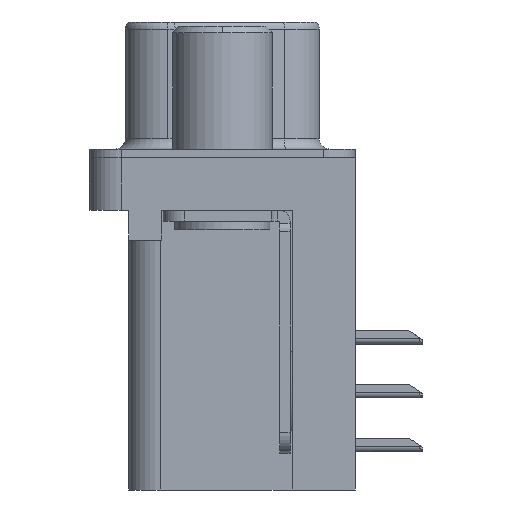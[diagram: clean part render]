
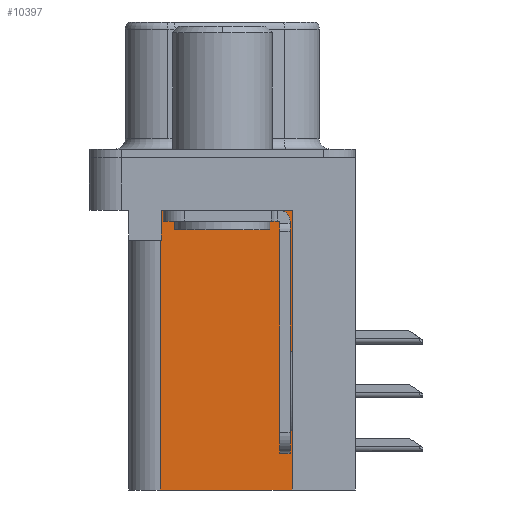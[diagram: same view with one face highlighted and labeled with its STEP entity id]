
A CAD part, left-side view. The second image highlights one B-rep face of the part: STEP entity #10397.
In plain terms, the highlighted planar face has unit normal (-1, 0, 0).
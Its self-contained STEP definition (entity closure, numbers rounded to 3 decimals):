
#514 = ORIENTED_EDGE ( 'NONE', *, *, #18524, .F. ) ;
#547 = DIRECTION ( 'NONE',  ( 0., 0., 1. ) ) ;
#1839 = ORIENTED_EDGE ( 'NONE', *, *, #3769, .T. ) ;
#2024 = CARTESIAN_POINT ( 'NONE',  ( 3.765, 2.895, -3.9 ) ) ;
#2810 = CARTESIAN_POINT ( 'NONE',  ( 3.765, -3.295, -2.5 ) ) ;
#2823 = CARTESIAN_POINT ( 'NONE',  ( 3.765, -3.295, -15.7 ) ) ;
#3165 = VERTEX_POINT ( 'NONE', #2810 ) ;
#3436 = VECTOR ( 'NONE', #25121, 1000. ) ;
#3769 = EDGE_CURVE ( 'NONE', #14060, #10398, #19271, .T. ) ;
#3882 = DIRECTION ( 'NONE',  ( 0., 0., -1. ) ) ;
#4667 = VERTEX_POINT ( 'NONE', #24077 ) ;
#4865 = VECTOR ( 'NONE', #547, 1000. ) ;
#5371 = VECTOR ( 'NONE', #24765, 1000. ) ;
#5867 = PLANE ( 'NONE',  #14750 ) ;
#6328 = EDGE_CURVE ( 'NONE', #3165, #4667, #23820, .T. ) ;
#6527 = ORIENTED_EDGE ( 'NONE', *, *, #6328, .T. ) ;
#6721 = VECTOR ( 'NONE', #19898, 1000. ) ;
#6760 = EDGE_CURVE ( 'NONE', #21742, #3165, #22274, .T. ) ;
#7051 = CARTESIAN_POINT ( 'NONE',  ( 3.765, 2.925, -15.7 ) ) ;
#7304 = VECTOR ( 'NONE', #22511, 1000. ) ;
#7611 = ORIENTED_EDGE ( 'NONE', *, *, #6760, .T. ) ;
#8208 = FACE_OUTER_BOUND ( 'NONE', #23082, .T. ) ;
#8701 = CARTESIAN_POINT ( 'NONE',  ( 3.765, -3.295, -15.7 ) ) ;
#9380 = VECTOR ( 'NONE', #25469, 1000. ) ;
#9716 = CARTESIAN_POINT ( 'NONE',  ( 3.765, -3.295, -15.7 ) ) ;
#10162 = EDGE_CURVE ( 'NONE', #21742, #13282, #22407, .T. ) ;
#10397 = ADVANCED_FACE ( 'NONE', ( #8208 ), #5867, .F. ) ;
#10398 = VERTEX_POINT ( 'NONE', #11663 ) ;
#10455 = CARTESIAN_POINT ( 'NONE',  ( 3.765, 2.925, -15.7 ) ) ;
#11663 = CARTESIAN_POINT ( 'NONE',  ( 3.765, 2.925, -3.9 ) ) ;
#13259 = CARTESIAN_POINT ( 'NONE',  ( 3.765, -3.295, -2.5 ) ) ;
#13282 = VERTEX_POINT ( 'NONE', #7051 ) ;
#14060 = VERTEX_POINT ( 'NONE', #14902 ) ;
#14750 = AXIS2_PLACEMENT_3D ( 'NONE', #9716, #15674, #3882 ) ;
#14902 = CARTESIAN_POINT ( 'NONE',  ( 3.765, 2.895, -3.9 ) ) ;
#15674 = DIRECTION ( 'NONE',  ( 1., 0., 0. ) ) ;
#17856 = EDGE_CURVE ( 'NONE', #4667, #14060, #22426, .T. ) ;
#18406 = ORIENTED_EDGE ( 'NONE', *, *, #17856, .T. ) ;
#18524 = EDGE_CURVE ( 'NONE', #13282, #10398, #20532, .T. ) ;
#19271 = LINE ( 'NONE', #23723, #9380 ) ;
#19898 = DIRECTION ( 'NONE',  ( 0., 0., -1. ) ) ;
#20532 = LINE ( 'NONE', #10455, #4865 ) ;
#21742 = VERTEX_POINT ( 'NONE', #2823 ) ;
#22274 = LINE ( 'NONE', #22783, #5371 ) ;
#22407 = LINE ( 'NONE', #8701, #7304 ) ;
#22426 = LINE ( 'NONE', #2024, #6721 ) ;
#22511 = DIRECTION ( 'NONE',  ( 0., 1., 0. ) ) ;
#22783 = CARTESIAN_POINT ( 'NONE',  ( 3.765, -3.295, -15.7 ) ) ;
#23082 = EDGE_LOOP ( 'NONE', ( #6527, #18406, #1839, #514, #23744, #7611 ) ) ;
#23723 = CARTESIAN_POINT ( 'NONE',  ( 3.765, 0., -3.9 ) ) ;
#23744 = ORIENTED_EDGE ( 'NONE', *, *, #10162, .F. ) ;
#23820 = LINE ( 'NONE', #13259, #3436 ) ;
#24077 = CARTESIAN_POINT ( 'NONE',  ( 3.765, 2.895, -2.5 ) ) ;
#24765 = DIRECTION ( 'NONE',  ( 0., 0., 1. ) ) ;
#25121 = DIRECTION ( 'NONE',  ( 0., 1., 0. ) ) ;
#25469 = DIRECTION ( 'NONE',  ( 0., 1., 0. ) ) ;
